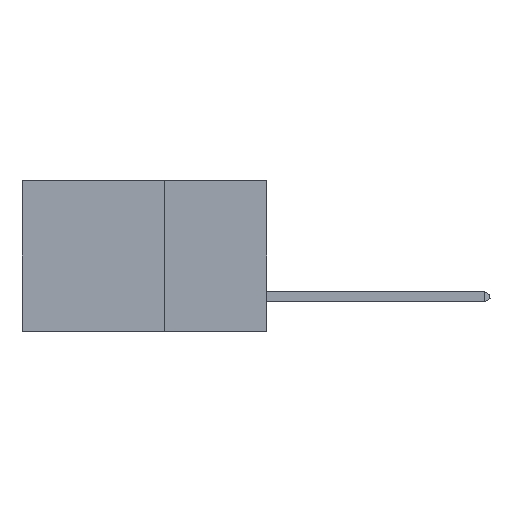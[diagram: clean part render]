
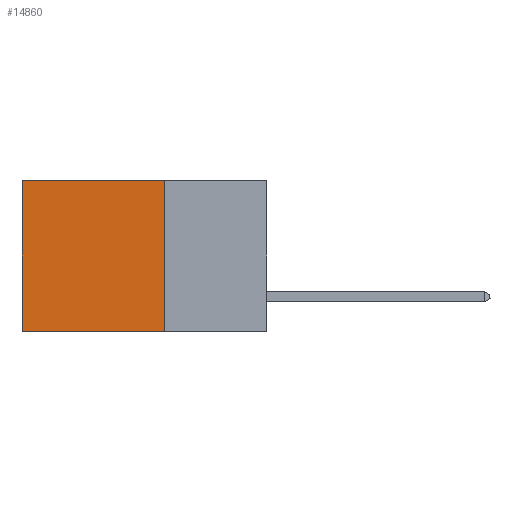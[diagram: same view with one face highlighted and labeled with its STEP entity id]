
A CAD part, left-side view. The second image highlights one B-rep face of the part: STEP entity #14860.
In plain terms, the highlighted planar face has unit normal (-1, 0, 0).
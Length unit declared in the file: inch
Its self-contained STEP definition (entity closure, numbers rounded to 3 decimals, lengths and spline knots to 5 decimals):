
#780 = LINE ( 'NONE', #2613, #2112 ) ;
#1327 = DIRECTION ( 'NONE',  ( 0., 0., -1. ) ) ;
#1731 = AXIS2_PLACEMENT_3D ( 'NONE', #8101, #7916, #10835 ) ;
#2112 = VECTOR ( 'NONE', #1327, 39.37008 ) ;
#2613 = CARTESIAN_POINT ( 'NONE',  ( 0.2875, 0.6, 0. ) ) ;
#2777 = ORIENTED_EDGE ( 'NONE', *, *, #11187, .T. ) ;
#3360 = FACE_OUTER_BOUND ( 'NONE', #11297, .T. ) ;
#4070 = VERTEX_POINT ( 'NONE', #8376 ) ;
#5220 = CARTESIAN_POINT ( 'NONE',  ( 0.2875, 0.25, 0. ) ) ;
#5747 = LINE ( 'NONE', #12095, #9894 ) ;
#6954 = CARTESIAN_POINT ( 'NONE',  ( 0.2875, 0.25, 0. ) ) ;
#7074 = DIRECTION ( 'NONE',  ( 0., 1., 0. ) ) ;
#7916 = DIRECTION ( 'NONE',  ( 1., 0., 0. ) ) ;
#8101 = CARTESIAN_POINT ( 'NONE',  ( 0.2875, 0.25, 0. ) ) ;
#8223 = ORIENTED_EDGE ( 'NONE', *, *, #14879, .F. ) ;
#8376 = CARTESIAN_POINT ( 'NONE',  ( 0.2875, 0.6, -0.37 ) ) ;
#9325 = VERTEX_POINT ( 'NONE', #16207 ) ;
#9894 = VECTOR ( 'NONE', #17680, 39.37008 ) ;
#10137 = EDGE_CURVE ( 'NONE', #9325, #4070, #13607, .T. ) ;
#10835 = DIRECTION ( 'NONE',  ( 0., 0., -1. ) ) ;
#11101 = ORIENTED_EDGE ( 'NONE', *, *, #13317, .T. ) ;
#11187 = EDGE_CURVE ( 'NONE', #13167, #16487, #15998, .T. ) ;
#11297 = EDGE_LOOP ( 'NONE', ( #11101, #14845, #8223, #2777 ) ) ;
#12095 = CARTESIAN_POINT ( 'NONE',  ( 0.2875, 0.25, 0. ) ) ;
#12425 = CARTESIAN_POINT ( 'NONE',  ( 0.2875, 0.25, -0.37 ) ) ;
#13167 = VERTEX_POINT ( 'NONE', #5220 ) ;
#13317 = EDGE_CURVE ( 'NONE', #16487, #4070, #780, .T. ) ;
#13595 = DIRECTION ( 'NONE',  ( 0., 1., 0. ) ) ;
#13607 = LINE ( 'NONE', #12425, #17550 ) ;
#14845 = ORIENTED_EDGE ( 'NONE', *, *, #10137, .F. ) ;
#14860 = ADVANCED_FACE ( 'NONE', ( #3360 ), #17863, .F. ) ;
#14879 = EDGE_CURVE ( 'NONE', #13167, #9325, #5747, .T. ) ;
#15112 = VECTOR ( 'NONE', #7074, 39.37008 ) ;
#15150 = CARTESIAN_POINT ( 'NONE',  ( 0.2875, 0.6, 0. ) ) ;
#15998 = LINE ( 'NONE', #6954, #15112 ) ;
#16207 = CARTESIAN_POINT ( 'NONE',  ( 0.2875, 0.25, -0.37 ) ) ;
#16487 = VERTEX_POINT ( 'NONE', #15150 ) ;
#17550 = VECTOR ( 'NONE', #13595, 39.37008 ) ;
#17680 = DIRECTION ( 'NONE',  ( 0., 0., -1. ) ) ;
#17863 = PLANE ( 'NONE',  #1731 ) ;
